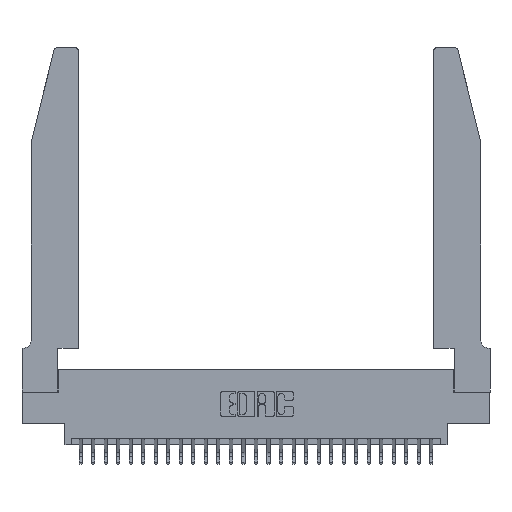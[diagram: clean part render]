
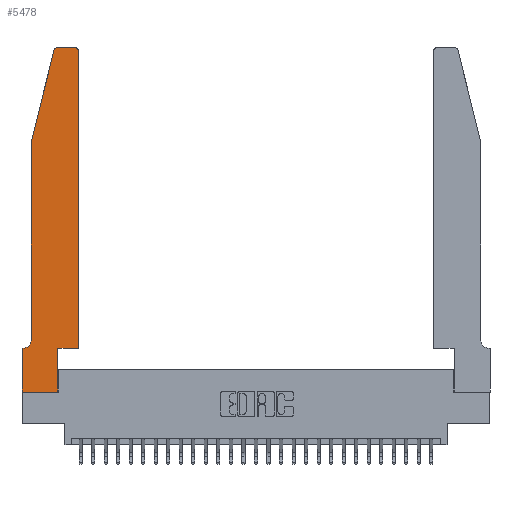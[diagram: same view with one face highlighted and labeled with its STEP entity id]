
A CAD part, top view. The second image highlights one B-rep face of the part: STEP entity #5478.
In plain terms, the highlighted planar face has unit normal (0, 0, 1).
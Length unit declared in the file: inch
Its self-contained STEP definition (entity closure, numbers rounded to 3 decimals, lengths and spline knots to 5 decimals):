
#756 = CIRCLE ( 'NONE', #24239, 0.03 ) ;
#855 = DIRECTION ( 'NONE',  ( 0., -1., 0. ) ) ;
#1111 = ORIENTED_EDGE ( 'NONE', *, *, #26925, .T. ) ;
#1153 = VECTOR ( 'NONE', #26805, 39.37008 ) ;
#1524 = LINE ( 'NONE', #25847, #19145 ) ;
#1567 = CIRCLE ( 'NONE', #17089, 0.03 ) ;
#1945 = CARTESIAN_POINT ( 'NONE',  ( 0.4505, 0.35, 0.37 ) ) ;
#2874 = AXIS2_PLACEMENT_3D ( 'NONE', #27370, #9500, #25304 ) ;
#2937 = EDGE_CURVE ( 'NONE', #4854, #24674, #756, .T. ) ;
#3136 = EDGE_CURVE ( 'NONE', #24674, #15884, #14616, .T. ) ;
#3193 = VECTOR ( 'NONE', #11156, 39.37008 ) ;
#3362 = LINE ( 'NONE', #17000, #21571 ) ;
#3830 = EDGE_CURVE ( 'NONE', #29438, #8925, #3362, .T. ) ;
#4155 = CARTESIAN_POINT ( 'NONE',  ( 0.2605, 2.75, 0.37 ) ) ;
#4435 = ORIENTED_EDGE ( 'NONE', *, *, #21516, .T. ) ;
#4793 = VERTEX_POINT ( 'NONE', #17936 ) ;
#4820 = EDGE_CURVE ( 'NONE', #23336, #29085, #26313, .T. ) ;
#4854 = VERTEX_POINT ( 'NONE', #22660 ) ;
#5478 = ADVANCED_FACE ( 'NONE', ( #15395 ), #18507, .T. ) ;
#5531 = LINE ( 'NONE', #10756, #17683 ) ;
#5966 = CARTESIAN_POINT ( 'NONE',  ( 0., 0.35, 0.37 ) ) ;
#6218 = CARTESIAN_POINT ( 'NONE',  ( 0.2865, 0.35, 0.37 ) ) ;
#6670 = VECTOR ( 'NONE', #27924, 39.37008 ) ;
#7088 = EDGE_CURVE ( 'NONE', #24483, #19219, #22309, .T. ) ;
#7411 = ORIENTED_EDGE ( 'NONE', *, *, #14763, .T. ) ;
#7751 = ORIENTED_EDGE ( 'NONE', *, *, #8496, .T. ) ;
#8139 = EDGE_CURVE ( 'NONE', #4793, #4854, #9951, .T. ) ;
#8496 = EDGE_CURVE ( 'NONE', #19219, #29438, #18777, .T. ) ;
#8519 = VECTOR ( 'NONE', #16993, 39.37008 ) ;
#8754 = CARTESIAN_POINT ( 'NONE',  ( 0.0755, 2., 0.37 ) ) ;
#8822 = ORIENTED_EDGE ( 'NONE', *, *, #8139, .T. ) ;
#8925 = VERTEX_POINT ( 'NONE', #17959 ) ;
#9020 = DIRECTION ( 'NONE',  ( 1., 0., 0. ) ) ;
#9232 = VECTOR ( 'NONE', #15654, 39.37008 ) ;
#9326 = DIRECTION ( 'NONE',  ( 0., 0., 1. ) ) ;
#9500 = DIRECTION ( 'NONE',  ( 0., 0., 1. ) ) ;
#9951 = LINE ( 'NONE', #4155, #9232 ) ;
#10756 = CARTESIAN_POINT ( 'NONE',  ( 0.4505, 0.35, 0.37 ) ) ;
#11156 = DIRECTION ( 'NONE',  ( 1., 0., 0. ) ) ;
#11704 = CARTESIAN_POINT ( 'NONE',  ( 0.284, 2.72, 0.37 ) ) ;
#12087 = ORIENTED_EDGE ( 'NONE', *, *, #4820, .T. ) ;
#12407 = CARTESIAN_POINT ( 'NONE',  ( 0.0055, 0.35, 0.37 ) ) ;
#12862 = CARTESIAN_POINT ( 'NONE',  ( 0.0755, 0.42, 0.37 ) ) ;
#13530 = LINE ( 'NONE', #8754, #1153 ) ;
#13648 = DIRECTION ( 'NONE',  ( 0., 0., -1. ) ) ;
#14005 = DIRECTION ( 'NONE',  ( 1., 0., 0. ) ) ;
#14481 = CARTESIAN_POINT ( 'NONE',  ( 0.0755, 0.35, 0.37 ) ) ;
#14570 = ORIENTED_EDGE ( 'NONE', *, *, #3830, .T. ) ;
#14616 = LINE ( 'NONE', #14772, #8519 ) ;
#14763 = EDGE_CURVE ( 'NONE', #19109, #4793, #1567, .T. ) ;
#14772 = CARTESIAN_POINT ( 'NONE',  ( 0.0755, 2., 0.37 ) ) ;
#15395 = FACE_OUTER_BOUND ( 'NONE', #25045, .T. ) ;
#15471 = EDGE_CURVE ( 'NONE', #15884, #24483, #13530, .T. ) ;
#15597 = ORIENTED_EDGE ( 'NONE', *, *, #2937, .T. ) ;
#15654 = DIRECTION ( 'NONE',  ( -1., 0., 0. ) ) ;
#15884 = VERTEX_POINT ( 'NONE', #23566 ) ;
#15905 = CARTESIAN_POINT ( 'NONE',  ( 0.25487, 2.72718, 0.37 ) ) ;
#16303 = ORIENTED_EDGE ( 'NONE', *, *, #3136, .T. ) ;
#16993 = DIRECTION ( 'NONE',  ( -0.239, -0.971, 0. ) ) ;
#17000 = CARTESIAN_POINT ( 'NONE',  ( 0., 0., 0.37 ) ) ;
#17089 = AXIS2_PLACEMENT_3D ( 'NONE', #22849, #9326, #25121 ) ;
#17354 = ORIENTED_EDGE ( 'NONE', *, *, #25949, .T. ) ;
#17514 = AXIS2_PLACEMENT_3D ( 'NONE', #27106, #13648, #29362 ) ;
#17683 = VECTOR ( 'NONE', #26509, 39.37008 ) ;
#17936 = CARTESIAN_POINT ( 'NONE',  ( 0.4205, 2.75, 0.37 ) ) ;
#17959 = CARTESIAN_POINT ( 'NONE',  ( 0., 0., 0.37 ) ) ;
#18236 = ORIENTED_EDGE ( 'NONE', *, *, #15471, .T. ) ;
#18507 = PLANE ( 'NONE',  #2874 ) ;
#18642 = VERTEX_POINT ( 'NONE', #23459 ) ;
#18777 = LINE ( 'NONE', #14481, #6670 ) ;
#19109 = VERTEX_POINT ( 'NONE', #25590 ) ;
#19145 = VECTOR ( 'NONE', #23594, 39.37008 ) ;
#19219 = VERTEX_POINT ( 'NONE', #12407 ) ;
#20703 = CARTESIAN_POINT ( 'NONE',  ( 0.4505, 0.35, 0.37 ) ) ;
#21516 = EDGE_CURVE ( 'NONE', #8925, #18642, #28114, .T. ) ;
#21571 = VECTOR ( 'NONE', #855, 39.37008 ) ;
#22309 = CIRCLE ( 'NONE', #17514, 0.07 ) ;
#22660 = CARTESIAN_POINT ( 'NONE',  ( 0.284, 2.75, 0.37 ) ) ;
#22849 = CARTESIAN_POINT ( 'NONE',  ( 0.4205, 2.72, 0.37 ) ) ;
#23336 = VERTEX_POINT ( 'NONE', #6218 ) ;
#23459 = CARTESIAN_POINT ( 'NONE',  ( 0.2865, 0., 0.37 ) ) ;
#23566 = CARTESIAN_POINT ( 'NONE',  ( 0.0755, 2., 0.37 ) ) ;
#23594 = DIRECTION ( 'NONE',  ( 0., 1., 0. ) ) ;
#24239 = AXIS2_PLACEMENT_3D ( 'NONE', #11704, #27447, #14005 ) ;
#24483 = VERTEX_POINT ( 'NONE', #12862 ) ;
#24674 = VERTEX_POINT ( 'NONE', #15905 ) ;
#25045 = EDGE_LOOP ( 'NONE', ( #8822, #15597, #16303, #18236, #25104, #7751, #14570, #4435, #17354, #12087, #1111, #7411 ) ) ;
#25104 = ORIENTED_EDGE ( 'NONE', *, *, #7088, .T. ) ;
#25121 = DIRECTION ( 'NONE',  ( 1., 0., 0. ) ) ;
#25304 = DIRECTION ( 'NONE',  ( 1., 0., 0. ) ) ;
#25590 = CARTESIAN_POINT ( 'NONE',  ( 0.4505, 2.72, 0.37 ) ) ;
#25631 = VECTOR ( 'NONE', #9020, 39.37008 ) ;
#25847 = CARTESIAN_POINT ( 'NONE',  ( 0.2865, 0.35, 0.37 ) ) ;
#25949 = EDGE_CURVE ( 'NONE', #18642, #23336, #1524, .T. ) ;
#26313 = LINE ( 'NONE', #1945, #25631 ) ;
#26509 = DIRECTION ( 'NONE',  ( 0., 1., 0. ) ) ;
#26805 = DIRECTION ( 'NONE',  ( 0., -1., 0. ) ) ;
#26925 = EDGE_CURVE ( 'NONE', #29085, #19109, #5531, .T. ) ;
#27106 = CARTESIAN_POINT ( 'NONE',  ( 0.0055, 0.42, 0.37 ) ) ;
#27370 = CARTESIAN_POINT ( 'NONE',  ( 0., 0.35, 0.37 ) ) ;
#27447 = DIRECTION ( 'NONE',  ( 0., 0., 1. ) ) ;
#27924 = DIRECTION ( 'NONE',  ( -1., 0., 0. ) ) ;
#28114 = LINE ( 'NONE', #29188, #3193 ) ;
#29085 = VERTEX_POINT ( 'NONE', #20703 ) ;
#29188 = CARTESIAN_POINT ( 'NONE',  ( 0., 0., 0.37 ) ) ;
#29362 = DIRECTION ( 'NONE',  ( -1., 0., 0. ) ) ;
#29438 = VERTEX_POINT ( 'NONE', #5966 ) ;
